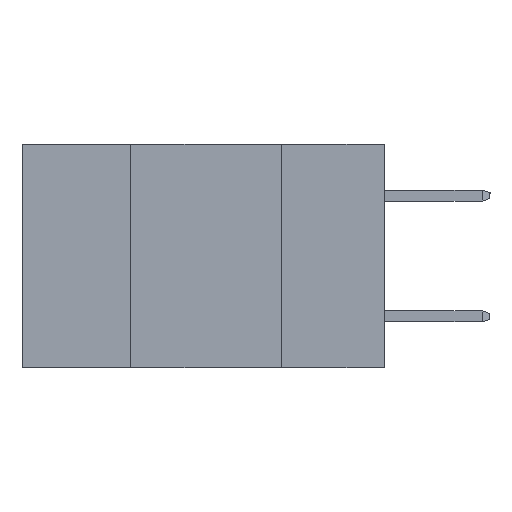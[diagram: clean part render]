
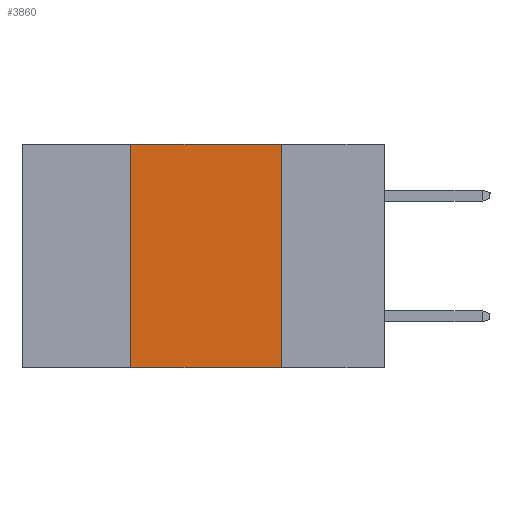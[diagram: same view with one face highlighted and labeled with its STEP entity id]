
A CAD part, left-side view. The second image highlights one B-rep face of the part: STEP entity #3860.
In plain terms, the highlighted planar face has unit normal (-1, 0, 0).
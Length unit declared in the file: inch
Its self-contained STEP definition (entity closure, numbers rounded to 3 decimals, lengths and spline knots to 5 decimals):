
#99 = CARTESIAN_POINT ( 'NONE',  ( 0., 0.6, 0. ) ) ;
#360 = CARTESIAN_POINT ( 'NONE',  ( 0., 0.42, -0.37 ) ) ;
#610 = CARTESIAN_POINT ( 'NONE',  ( 0., 0.42, -0.37 ) ) ;
#641 = PLANE ( 'NONE',  #3837 ) ;
#957 = EDGE_LOOP ( 'NONE', ( #7189, #3484, #7719, #8500 ) ) ;
#1864 = CARTESIAN_POINT ( 'NONE',  ( 0., 0.6, 0. ) ) ;
#1871 = VECTOR ( 'NONE', #4710, 39.37008 ) ;
#3379 = VERTEX_POINT ( 'NONE', #610 ) ;
#3484 = ORIENTED_EDGE ( 'NONE', *, *, #12914, .F. ) ;
#3756 = EDGE_CURVE ( 'NONE', #3379, #5961, #12226, .T. ) ;
#3837 = AXIS2_PLACEMENT_3D ( 'NONE', #1864, #12437, #3928 ) ;
#3860 = ADVANCED_FACE ( 'NONE', ( #9376 ), #641, .F. ) ;
#3928 = DIRECTION ( 'NONE',  ( 0., 0., -1. ) ) ;
#3973 = VECTOR ( 'NONE', #9767, 39.37008 ) ;
#4495 = VECTOR ( 'NONE', #6846, 39.37008 ) ;
#4710 = DIRECTION ( 'NONE',  ( 0., 0., 1. ) ) ;
#4730 = DIRECTION ( 'NONE',  ( 0., 0., -1. ) ) ;
#4798 = VERTEX_POINT ( 'NONE', #6951 ) ;
#5222 = EDGE_CURVE ( 'NONE', #4798, #5961, #7001, .T. ) ;
#5576 = CARTESIAN_POINT ( 'NONE',  ( 0., 0.17, -0.37 ) ) ;
#5961 = VERTEX_POINT ( 'NONE', #5576 ) ;
#6846 = DIRECTION ( 'NONE',  ( 0., -1., 0. ) ) ;
#6951 = CARTESIAN_POINT ( 'NONE',  ( 0., 0.17, 0. ) ) ;
#7001 = LINE ( 'NONE', #9051, #7718 ) ;
#7189 = ORIENTED_EDGE ( 'NONE', *, *, #5222, .F. ) ;
#7718 = VECTOR ( 'NONE', #4730, 39.37008 ) ;
#7719 = ORIENTED_EDGE ( 'NONE', *, *, #9643, .F. ) ;
#7902 = CARTESIAN_POINT ( 'NONE',  ( 0., 0.6, -0.37 ) ) ;
#8500 = ORIENTED_EDGE ( 'NONE', *, *, #3756, .T. ) ;
#9051 = CARTESIAN_POINT ( 'NONE',  ( 0., 0.17, -0.37 ) ) ;
#9278 = VERTEX_POINT ( 'NONE', #9810 ) ;
#9376 = FACE_OUTER_BOUND ( 'NONE', #957, .T. ) ;
#9643 = EDGE_CURVE ( 'NONE', #3379, #9278, #10095, .T. ) ;
#9767 = DIRECTION ( 'NONE',  ( 0., -1., 0. ) ) ;
#9810 = CARTESIAN_POINT ( 'NONE',  ( 0., 0.42, 0. ) ) ;
#9907 = LINE ( 'NONE', #99, #3973 ) ;
#10095 = LINE ( 'NONE', #360, #1871 ) ;
#12226 = LINE ( 'NONE', #7902, #4495 ) ;
#12437 = DIRECTION ( 'NONE',  ( 1., 0., 0. ) ) ;
#12914 = EDGE_CURVE ( 'NONE', #9278, #4798, #9907, .T. ) ;
